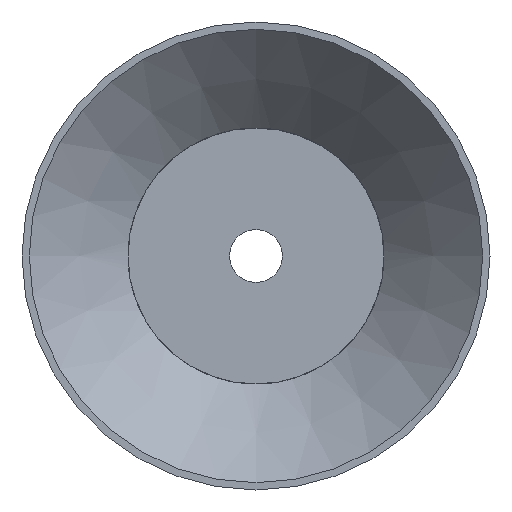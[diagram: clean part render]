
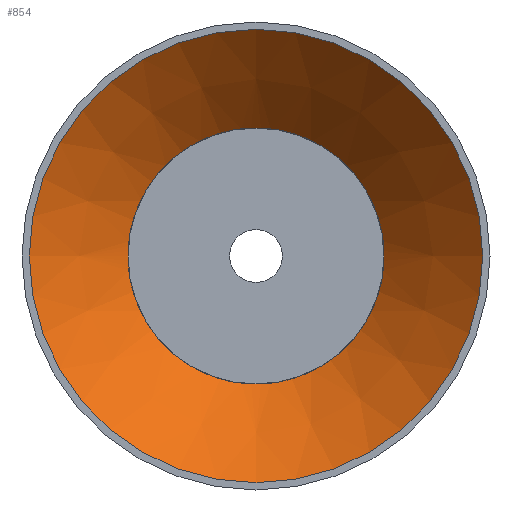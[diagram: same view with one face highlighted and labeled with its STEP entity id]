
A CAD part, front view. The second image highlights one B-rep face of the part: STEP entity #854.
In plain terms, the highlighted conical face has half-angle 44.2 degrees and reference radius 30.725 mm.
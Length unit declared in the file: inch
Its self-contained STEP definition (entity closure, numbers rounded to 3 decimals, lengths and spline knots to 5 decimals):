
#118=(
BOUNDED_CURVE()
B_SPLINE_CURVE(2,(#1162,#1163,#1164),.UNSPECIFIED.,.F.,.F.)
B_SPLINE_CURVE_WITH_KNOTS((3,3),(0.,0.02357),.UNSPECIFIED.)
CURVE()
GEOMETRIC_REPRESENTATION_ITEM()
RATIONAL_B_SPLINE_CURVE((1.,1.,1.))
REPRESENTATION_ITEM('')
);
#119=(
BOUNDED_CURVE()
B_SPLINE_CURVE(2,(#1166,#1167,#1168),.UNSPECIFIED.,.F.,.F.)
B_SPLINE_CURVE_WITH_KNOTS((3,3),(0.84814,0.87172),
 .UNSPECIFIED.)
CURVE()
GEOMETRIC_REPRESENTATION_ITEM()
RATIONAL_B_SPLINE_CURVE((1.,1.,1.))
REPRESENTATION_ITEM('')
);
#120=(
BOUNDED_CURVE()
B_SPLINE_CURVE(2,(#1171,#1172,#1173),.UNSPECIFIED.,.F.,.F.)
B_SPLINE_CURVE_WITH_KNOTS((3,3),(0.,0.02357),.UNSPECIFIED.)
CURVE()
GEOMETRIC_REPRESENTATION_ITEM()
RATIONAL_B_SPLINE_CURVE((1.,1.,1.))
REPRESENTATION_ITEM('')
);
#121=(
BOUNDED_CURVE()
B_SPLINE_CURVE(2,(#1175,#1176,#1177),.UNSPECIFIED.,.F.,.F.)
B_SPLINE_CURVE_WITH_KNOTS((3,3),(0.84824,0.87181),
 .UNSPECIFIED.)
CURVE()
GEOMETRIC_REPRESENTATION_ITEM()
RATIONAL_B_SPLINE_CURVE((1.,1.,1.))
REPRESENTATION_ITEM('')
);
#122=(
BOUNDED_CURVE()
B_SPLINE_CURVE(2,(#1181,#1182,#1183),.UNSPECIFIED.,.F.,.F.)
B_SPLINE_CURVE_WITH_KNOTS((3,3),(0.,0.02357),.UNSPECIFIED.)
CURVE()
GEOMETRIC_REPRESENTATION_ITEM()
RATIONAL_B_SPLINE_CURVE((1.,1.,1.))
REPRESENTATION_ITEM('')
);
#123=(
BOUNDED_CURVE()
B_SPLINE_CURVE(2,(#1187,#1188,#1189),.UNSPECIFIED.,.F.,.F.)
B_SPLINE_CURVE_WITH_KNOTS((3,3),(0.84823,0.87181),
 .UNSPECIFIED.)
CURVE()
GEOMETRIC_REPRESENTATION_ITEM()
RATIONAL_B_SPLINE_CURVE((1.,1.,1.))
REPRESENTATION_ITEM('')
);
#124=(
BOUNDED_CURVE()
B_SPLINE_CURVE(2,(#1192,#1193,#1194),.UNSPECIFIED.,.F.,.F.)
B_SPLINE_CURVE_WITH_KNOTS((3,3),(0.,0.02357),.UNSPECIFIED.)
CURVE()
GEOMETRIC_REPRESENTATION_ITEM()
RATIONAL_B_SPLINE_CURVE((1.,1.,1.))
REPRESENTATION_ITEM('')
);
#125=(
BOUNDED_CURVE()
B_SPLINE_CURVE(2,(#1196,#1197,#1198),.UNSPECIFIED.,.F.,.F.)
B_SPLINE_CURVE_WITH_KNOTS((3,3),(0.84802,0.87159),
 .UNSPECIFIED.)
CURVE()
GEOMETRIC_REPRESENTATION_ITEM()
RATIONAL_B_SPLINE_CURVE((1.,1.,1.))
REPRESENTATION_ITEM('')
);
#127=CONICAL_SURFACE('',#914,1.20964,0.771);
#132=FACE_OUTER_BOUND('',#172,.T.);
#172=EDGE_LOOP('',(#565,#566,#567,#568,#569,#570,#571,#572,#573,#574,#575,
#576,#577,#578,#579,#580,#581,#582,#583,#584,#585));
#213=CIRCLE('',#907,0.86927);
#215=CIRCLE('',#910,0.86927);
#216=CIRCLE('',#912,0.86927);
#218=CIRCLE('',#915,1.55);
#219=CIRCLE('',#916,0.875);
#220=CIRCLE('',#917,0.875);
#221=CIRCLE('',#918,0.875);
#222=CIRCLE('',#919,0.86927);
#223=CIRCLE('',#920,0.875);
#224=CIRCLE('',#921,0.875);
#225=CIRCLE('',#922,1.55);
#254=LINE('',#1159,#284);
#284=VECTOR('',#998,1.20964);
#309=VERTEX_POINT('',#1129);
#311=VERTEX_POINT('',#1133);
#313=VERTEX_POINT('',#1138);
#315=VERTEX_POINT('',#1142);
#316=VERTEX_POINT('',#1146);
#318=VERTEX_POINT('',#1149);
#320=VERTEX_POINT('',#1155);
#321=VERTEX_POINT('',#1156);
#322=VERTEX_POINT('',#1158);
#323=VERTEX_POINT('',#1160);
#324=VERTEX_POINT('',#1165);
#325=VERTEX_POINT('',#1169);
#326=VERTEX_POINT('',#1174);
#327=VERTEX_POINT('',#1178);
#328=VERTEX_POINT('',#1180);
#329=VERTEX_POINT('',#1184);
#330=VERTEX_POINT('',#1186);
#331=VERTEX_POINT('',#1190);
#332=VERTEX_POINT('',#1195);
#411=EDGE_CURVE('',#311,#309,#213,.T.);
#415=EDGE_CURVE('',#315,#313,#215,.T.);
#417=EDGE_CURVE('',#316,#318,#216,.T.);
#420=EDGE_CURVE('',#320,#321,#218,.T.);
#421=EDGE_CURVE('',#321,#322,#254,.T.);
#422=EDGE_CURVE('',#323,#322,#219,.T.);
#423=EDGE_CURVE('',#309,#323,#118,.T.);
#424=EDGE_CURVE('',#324,#311,#119,.T.);
#425=EDGE_CURVE('',#325,#324,#220,.T.);
#426=EDGE_CURVE('',#318,#325,#120,.T.);
#427=EDGE_CURVE('',#326,#316,#121,.T.);
#428=EDGE_CURVE('',#327,#326,#221,.T.);
#429=EDGE_CURVE('',#328,#327,#122,.T.);
#430=EDGE_CURVE('',#329,#328,#222,.T.);
#431=EDGE_CURVE('',#330,#329,#123,.T.);
#432=EDGE_CURVE('',#331,#330,#223,.T.);
#433=EDGE_CURVE('',#313,#331,#124,.T.);
#434=EDGE_CURVE('',#332,#315,#125,.T.);
#435=EDGE_CURVE('',#322,#332,#224,.T.);
#436=EDGE_CURVE('',#321,#320,#225,.T.);
#565=ORIENTED_EDGE('',*,*,#420,.T.);
#566=ORIENTED_EDGE('',*,*,#421,.T.);
#567=ORIENTED_EDGE('',*,*,#422,.F.);
#568=ORIENTED_EDGE('',*,*,#423,.F.);
#569=ORIENTED_EDGE('',*,*,#411,.F.);
#570=ORIENTED_EDGE('',*,*,#424,.F.);
#571=ORIENTED_EDGE('',*,*,#425,.F.);
#572=ORIENTED_EDGE('',*,*,#426,.F.);
#573=ORIENTED_EDGE('',*,*,#417,.F.);
#574=ORIENTED_EDGE('',*,*,#427,.F.);
#575=ORIENTED_EDGE('',*,*,#428,.F.);
#576=ORIENTED_EDGE('',*,*,#429,.F.);
#577=ORIENTED_EDGE('',*,*,#430,.F.);
#578=ORIENTED_EDGE('',*,*,#431,.F.);
#579=ORIENTED_EDGE('',*,*,#432,.F.);
#580=ORIENTED_EDGE('',*,*,#433,.F.);
#581=ORIENTED_EDGE('',*,*,#415,.F.);
#582=ORIENTED_EDGE('',*,*,#434,.F.);
#583=ORIENTED_EDGE('',*,*,#435,.F.);
#584=ORIENTED_EDGE('',*,*,#421,.F.);
#585=ORIENTED_EDGE('',*,*,#436,.T.);
#854=ADVANCED_FACE('',(#132),#127,.F.);
#907=AXIS2_PLACEMENT_3D('',#1135,#976,#977);
#910=AXIS2_PLACEMENT_3D('',#1144,#984,#985);
#912=AXIS2_PLACEMENT_3D('',#1150,#989,#990);
#914=AXIS2_PLACEMENT_3D('',#1154,#994,#995);
#915=AXIS2_PLACEMENT_3D('',#1157,#996,#997);
#916=AXIS2_PLACEMENT_3D('',#1161,#999,#1000);
#917=AXIS2_PLACEMENT_3D('',#1170,#1001,#1002);
#918=AXIS2_PLACEMENT_3D('',#1179,#1003,#1004);
#919=AXIS2_PLACEMENT_3D('',#1185,#1005,#1006);
#920=AXIS2_PLACEMENT_3D('',#1191,#1007,#1008);
#921=AXIS2_PLACEMENT_3D('',#1199,#1009,#1010);
#922=AXIS2_PLACEMENT_3D('',#1200,#1011,#1012);
#976=DIRECTION('center_axis',(0.,-1.,0.));
#977=DIRECTION('ref_axis',(1.,0.,0.));
#984=DIRECTION('center_axis',(0.,-1.,0.));
#985=DIRECTION('ref_axis',(1.,0.,0.));
#989=DIRECTION('center_axis',(0.,-1.,0.));
#990=DIRECTION('ref_axis',(1.,0.,0.));
#994=DIRECTION('center_axis',(0.,-1.,0.));
#995=DIRECTION('ref_axis',(1.,0.,0.));
#996=DIRECTION('center_axis',(0.,-1.,0.));
#997=DIRECTION('ref_axis',(1.,0.,0.));
#998=DIRECTION('',(0.697,0.717,0.));
#999=DIRECTION('center_axis',(0.,-1.,0.));
#1000=DIRECTION('ref_axis',(1.,0.,0.));
#1001=DIRECTION('center_axis',(0.,-1.,0.));
#1002=DIRECTION('ref_axis',(1.,0.,0.));
#1003=DIRECTION('center_axis',(0.,-1.,0.));
#1004=DIRECTION('ref_axis',(1.,0.,0.));
#1005=DIRECTION('center_axis',(0.,-1.,0.));
#1006=DIRECTION('ref_axis',(1.,0.,0.));
#1007=DIRECTION('center_axis',(0.,-1.,0.));
#1008=DIRECTION('ref_axis',(1.,0.,0.));
#1009=DIRECTION('center_axis',(0.,-1.,0.));
#1010=DIRECTION('ref_axis',(1.,0.,0.));
#1011=DIRECTION('center_axis',(0.,-1.,0.));
#1012=DIRECTION('ref_axis',(1.,0.,0.));
#1129=CARTESIAN_POINT('',(-0.8635,0.7,0.1));
#1133=CARTESIAN_POINT('',(-0.10004,0.7,0.8635));
#1135=CARTESIAN_POINT('Origin',(0.,0.7,0.));
#1138=CARTESIAN_POINT('',(-0.1,0.7,-0.8635));
#1142=CARTESIAN_POINT('',(-0.86348,0.7,-0.10016));
#1144=CARTESIAN_POINT('Origin',(0.,0.7,0.));
#1146=CARTESIAN_POINT('',(0.86351,0.7,0.09995));
#1149=CARTESIAN_POINT('',(0.1,0.7,0.8635));
#1150=CARTESIAN_POINT('Origin',(0.,0.7,0.));
#1154=CARTESIAN_POINT('Origin',(0.,0.35,
0.));
#1155=CARTESIAN_POINT('',(1.55,0.,0.));
#1156=CARTESIAN_POINT('',(-1.55,0.,0.));
#1157=CARTESIAN_POINT('Origin',(0.,0.,
0.));
#1158=CARTESIAN_POINT('',(-0.875,0.69411,0.));
#1159=CARTESIAN_POINT('',(-1.20964,0.35,0.));
#1160=CARTESIAN_POINT('',(-0.86927,0.69411,0.1));
#1161=CARTESIAN_POINT('Origin',(0.,0.69411,0.));
#1162=CARTESIAN_POINT('Ctrl Pts',(-0.8635,0.7,
0.1));
#1163=CARTESIAN_POINT('Ctrl Pts',(-0.86638,0.69707,
0.1));
#1164=CARTESIAN_POINT('Ctrl Pts',(-0.86927,0.69411,
0.1));
#1165=CARTESIAN_POINT('',(-0.10004,0.69411,0.86926));
#1166=CARTESIAN_POINT('Ctrl Pts',(-0.10004,0.69411,
0.86926));
#1167=CARTESIAN_POINT('Ctrl Pts',(-0.10004,0.69707,0.86637));
#1168=CARTESIAN_POINT('Ctrl Pts',(-0.10004,0.7,
0.8635));
#1169=CARTESIAN_POINT('',(0.1,0.69411,0.86927));
#1170=CARTESIAN_POINT('Origin',(0.,0.69411,0.));
#1171=CARTESIAN_POINT('Ctrl Pts',(0.1,0.7,0.8635));
#1172=CARTESIAN_POINT('Ctrl Pts',(0.1,0.69707,0.86638));
#1173=CARTESIAN_POINT('Ctrl Pts',(0.1,0.69411,0.86927));
#1174=CARTESIAN_POINT('',(0.86927,0.69411,0.09995));
#1175=CARTESIAN_POINT('Ctrl Pts',(0.86927,0.69411,0.09995));
#1176=CARTESIAN_POINT('Ctrl Pts',(0.86638,0.69707,0.09995));
#1177=CARTESIAN_POINT('Ctrl Pts',(0.86351,0.7,0.09995));
#1178=CARTESIAN_POINT('',(0.86927,0.69411,-0.1));
#1179=CARTESIAN_POINT('Origin',(0.,0.69411,0.));
#1180=CARTESIAN_POINT('',(0.8635,0.7,-0.1));
#1181=CARTESIAN_POINT('Ctrl Pts',(0.8635,0.7,-0.1));
#1182=CARTESIAN_POINT('Ctrl Pts',(0.86638,0.69707,-0.1));
#1183=CARTESIAN_POINT('Ctrl Pts',(0.86927,0.69411,-0.1));
#1184=CARTESIAN_POINT('',(0.09995,0.7,-0.86351));
#1185=CARTESIAN_POINT('Origin',(0.,0.7,0.));
#1186=CARTESIAN_POINT('',(0.09995,0.69411,-0.86927));
#1187=CARTESIAN_POINT('Ctrl Pts',(0.09995,0.69411,
-0.86927));
#1188=CARTESIAN_POINT('Ctrl Pts',(0.09995,0.69707,
-0.86638));
#1189=CARTESIAN_POINT('Ctrl Pts',(0.09995,0.7,
-0.86351));
#1190=CARTESIAN_POINT('',(-0.1,0.69411,-0.86927));
#1191=CARTESIAN_POINT('Origin',(0.,0.69411,0.));
#1192=CARTESIAN_POINT('Ctrl Pts',(-0.1,0.7,
-0.8635));
#1193=CARTESIAN_POINT('Ctrl Pts',(-0.1,0.69707,
-0.86638));
#1194=CARTESIAN_POINT('Ctrl Pts',(-0.1,0.69411,
-0.86927));
#1195=CARTESIAN_POINT('',(-0.86925,0.69411,-0.10017));
#1196=CARTESIAN_POINT('Ctrl Pts',(-0.86925,0.69411,
-0.10017));
#1197=CARTESIAN_POINT('Ctrl Pts',(-0.86636,0.69707,
-0.10017));
#1198=CARTESIAN_POINT('Ctrl Pts',(-0.86348,0.7,
-0.10016));
#1199=CARTESIAN_POINT('Origin',(0.,0.69411,0.));
#1200=CARTESIAN_POINT('Origin',(0.,0.,
0.));
